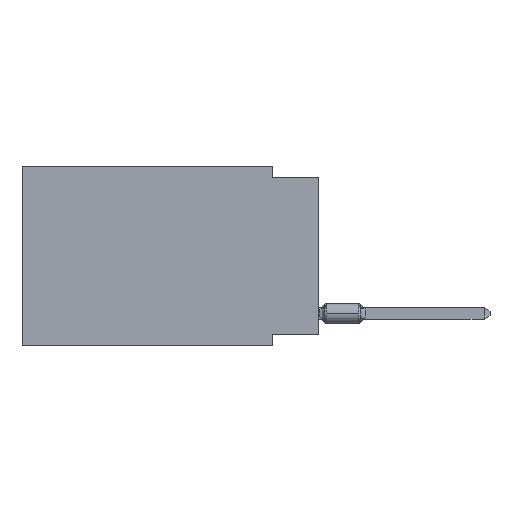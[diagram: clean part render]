
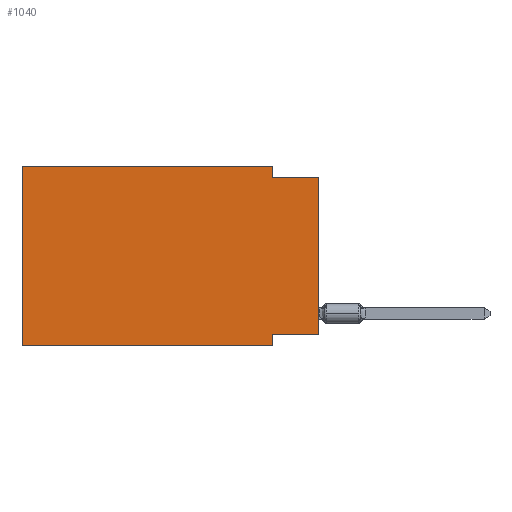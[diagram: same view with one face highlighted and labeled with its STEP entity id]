
A CAD part, left-side view. The second image highlights one B-rep face of the part: STEP entity #1040.
In plain terms, the highlighted planar face has unit normal (-1, 0, 0).
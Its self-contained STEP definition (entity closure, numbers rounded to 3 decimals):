
#51 = EDGE_CURVE ( 'NONE', #24462, #6918, #19225, .T. ) ;
#71 = DIRECTION ( 'NONE',  ( 0., -1., 0. ) ) ;
#165 = CARTESIAN_POINT ( 'NONE',  ( 0., 16.383, -9.906 ) ) ;
#1040 = ADVANCED_FACE ( 'NONE', ( #5338 ), #15121, .F. ) ;
#1059 = ORIENTED_EDGE ( 'NONE', *, *, #15167, .F. ) ;
#1583 = CARTESIAN_POINT ( 'NONE',  ( 0., 2.54, -9.271 ) ) ;
#1657 = LINE ( 'NONE', #5325, #9118 ) ;
#2044 = VECTOR ( 'NONE', #12572, 1000. ) ;
#3442 = DIRECTION ( 'NONE',  ( 0., 0., -1. ) ) ;
#3573 = CARTESIAN_POINT ( 'NONE',  ( 0., 16.383, 0. ) ) ;
#5325 = CARTESIAN_POINT ( 'NONE',  ( 0., 2.54, -9.906 ) ) ;
#5338 = FACE_OUTER_BOUND ( 'NONE', #17739, .T. ) ;
#6222 = DIRECTION ( 'NONE',  ( 0., 0., 1. ) ) ;
#6228 = CARTESIAN_POINT ( 'NONE',  ( 0., 16.383, 0. ) ) ;
#6517 = CARTESIAN_POINT ( 'NONE',  ( 0., 0., -9.271 ) ) ;
#6918 = VERTEX_POINT ( 'NONE', #7503 ) ;
#7236 = ORIENTED_EDGE ( 'NONE', *, *, #15001, .F. ) ;
#7503 = CARTESIAN_POINT ( 'NONE',  ( 0., 2.54, 0. ) ) ;
#7572 = EDGE_CURVE ( 'NONE', #20091, #24462, #16912, .T. ) ;
#7814 = EDGE_CURVE ( 'NONE', #8647, #19573, #15744, .T. ) ;
#8647 = VERTEX_POINT ( 'NONE', #6517 ) ;
#8730 = VECTOR ( 'NONE', #6222, 1000. ) ;
#9118 = VECTOR ( 'NONE', #14863, 1000. ) ;
#9171 = ORIENTED_EDGE ( 'NONE', *, *, #7814, .T. ) ;
#9756 = ORIENTED_EDGE ( 'NONE', *, *, #18116, .F. ) ;
#11381 = CARTESIAN_POINT ( 'NONE',  ( 0., 16.383, -9.906 ) ) ;
#11385 = DIRECTION ( 'NONE',  ( 0., -1., 0. ) ) ;
#11967 = VECTOR ( 'NONE', #24691, 1000. ) ;
#12572 = DIRECTION ( 'NONE',  ( 0., 0., -1. ) ) ;
#13836 = DIRECTION ( 'NONE',  ( 0., 1., 0. ) ) ;
#14191 = VECTOR ( 'NONE', #13836, 1000. ) ;
#14863 = DIRECTION ( 'NONE',  ( 0., 0., -1. ) ) ;
#15001 = EDGE_CURVE ( 'NONE', #8647, #23779, #18919, .T. ) ;
#15121 = PLANE ( 'NONE',  #20794 ) ;
#15167 = EDGE_CURVE ( 'NONE', #6918, #16491, #20180, .T. ) ;
#15232 = VECTOR ( 'NONE', #19442, 1000. ) ;
#15640 = LINE ( 'NONE', #165, #15232 ) ;
#15744 = LINE ( 'NONE', #23906, #8730 ) ;
#16491 = VERTEX_POINT ( 'NONE', #23160 ) ;
#16824 = CARTESIAN_POINT ( 'NONE',  ( 0., 16.383, 0. ) ) ;
#16912 = LINE ( 'NONE', #22394, #11967 ) ;
#17328 = LINE ( 'NONE', #21645, #19230 ) ;
#17739 = EDGE_LOOP ( 'NONE', ( #9171, #20970, #1059, #18639, #19677, #18298, #9756, #7236 ) ) ;
#18116 = EDGE_CURVE ( 'NONE', #23779, #20392, #1657, .T. ) ;
#18262 = CARTESIAN_POINT ( 'NONE',  ( 0., 2.54, 0. ) ) ;
#18298 = ORIENTED_EDGE ( 'NONE', *, *, #22275, .T. ) ;
#18639 = ORIENTED_EDGE ( 'NONE', *, *, #51, .F. ) ;
#18699 = VECTOR ( 'NONE', #11385, 1000. ) ;
#18919 = LINE ( 'NONE', #21331, #14191 ) ;
#19225 = LINE ( 'NONE', #16824, #18699 ) ;
#19230 = VECTOR ( 'NONE', #71, 1000. ) ;
#19442 = DIRECTION ( 'NONE',  ( 0., -1., 0. ) ) ;
#19573 = VERTEX_POINT ( 'NONE', #22115 ) ;
#19677 = ORIENTED_EDGE ( 'NONE', *, *, #7572, .F. ) ;
#20091 = VERTEX_POINT ( 'NONE', #11381 ) ;
#20180 = LINE ( 'NONE', #18262, #2044 ) ;
#20392 = VERTEX_POINT ( 'NONE', #23306 ) ;
#20794 = AXIS2_PLACEMENT_3D ( 'NONE', #3573, #20956, #3442 ) ;
#20956 = DIRECTION ( 'NONE',  ( 1., 0., 0. ) ) ;
#20970 = ORIENTED_EDGE ( 'NONE', *, *, #23491, .F. ) ;
#21331 = CARTESIAN_POINT ( 'NONE',  ( 0., 0., -9.271 ) ) ;
#21645 = CARTESIAN_POINT ( 'NONE',  ( 0., 0., -0.635 ) ) ;
#22115 = CARTESIAN_POINT ( 'NONE',  ( 0., 0., -0.635 ) ) ;
#22275 = EDGE_CURVE ( 'NONE', #20091, #20392, #15640, .T. ) ;
#22394 = CARTESIAN_POINT ( 'NONE',  ( 0., 16.383, 0. ) ) ;
#23160 = CARTESIAN_POINT ( 'NONE',  ( 0., 2.54, -0.635 ) ) ;
#23306 = CARTESIAN_POINT ( 'NONE',  ( 0., 2.54, -9.906 ) ) ;
#23491 = EDGE_CURVE ( 'NONE', #16491, #19573, #17328, .T. ) ;
#23779 = VERTEX_POINT ( 'NONE', #1583 ) ;
#23906 = CARTESIAN_POINT ( 'NONE',  ( 0., 0., 0. ) ) ;
#24462 = VERTEX_POINT ( 'NONE', #6228 ) ;
#24691 = DIRECTION ( 'NONE',  ( 0., 0., 1. ) ) ;
